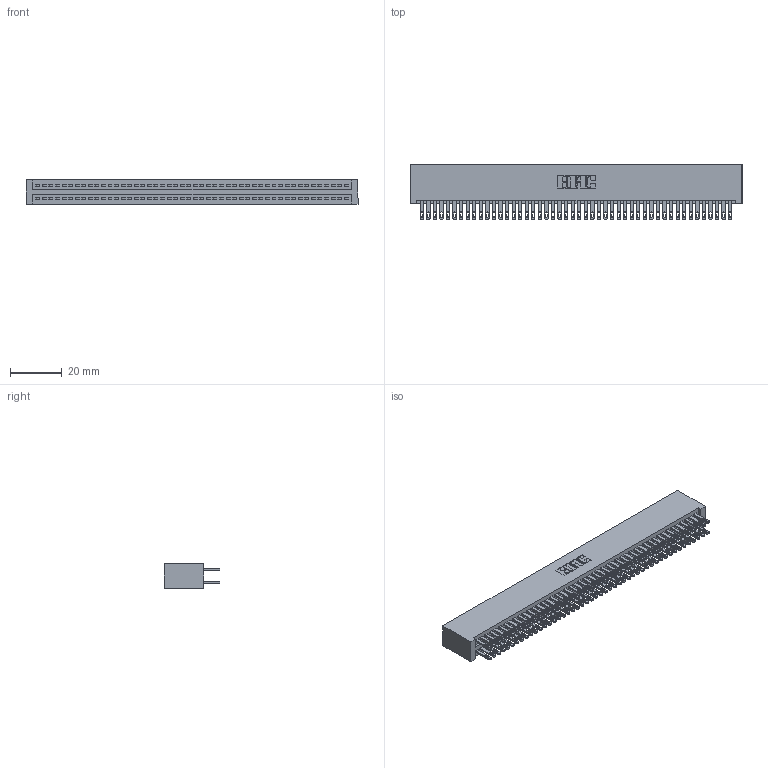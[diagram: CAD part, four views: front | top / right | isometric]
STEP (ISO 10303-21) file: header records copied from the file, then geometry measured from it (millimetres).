
FILE_DESCRIPTION (( 'STEP AP203' ), '1' );
FILE_NAME ('345-096-500-201.STEP', '2019-11-02T06:26:45', ( '' ), ( '' ), 'SwSTEP 2.0', 'SolidWorks 2016', '' );
FILE_SCHEMA (( 'CONFIG_CONTROL_DESIGN' ));
Length unit declared in the file: inch
Products named in the file (3): 345 Part_No Mounting Lugs; 345-292-001_345-293-100; 345-096-500-201
Assembly tree (97 placements, depth 2):
  345-096-500-201
    345 Part_No Mounting Lugs
    345-292-001_345-293-100  x96
Bounding box: 128.52 x 21.51 x 9.4 mm (x, y, z)
Volume: 13449.9 mm3; surface area: 21279.9 mm2
Topology: 97 solids, 97 shells, 4534 faces, 13853 edges, 9234 vertices
Faces by surface type: plane 2668, cylinder 1866
Entity records: 36507 total; most frequent: CARTESIAN_POINT 6112, ORIENTED_EDGE 6046, DIRECTION 5379, EDGE_CURVE 3023, VECTOR 2703, LINE 2703, VERTEX_POINT 2014, AXIS2_PLACEMENT_3D 1338
